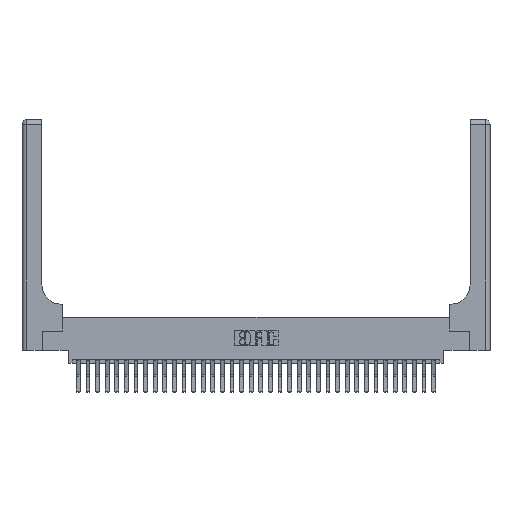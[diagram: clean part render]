
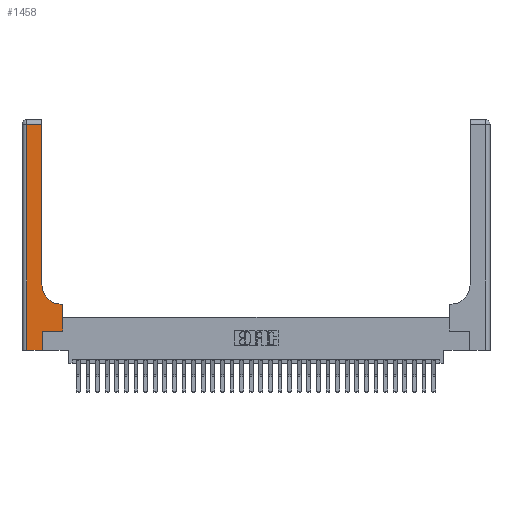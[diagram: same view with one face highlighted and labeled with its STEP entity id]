
A CAD part, top view. The second image highlights one B-rep face of the part: STEP entity #1458.
In plain terms, the highlighted planar face has unit normal (0, 0, 1).
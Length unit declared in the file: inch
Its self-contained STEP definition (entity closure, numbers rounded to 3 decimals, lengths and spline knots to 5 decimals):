
#541 = LINE ( 'NONE', #20445, #6170 ) ;
#696 = EDGE_CURVE ( 'NONE', #22260, #21338, #13939, .T. ) ;
#1458 = ADVANCED_FACE ( 'NONE', ( #4975 ), #24261, .F. ) ;
#2265 = LINE ( 'NONE', #23883, #15712 ) ;
#3300 = VECTOR ( 'NONE', #7871, 39.37008 ) ;
#3541 = EDGE_CURVE ( 'NONE', #21365, #20497, #11126, .T. ) ;
#3670 = CARTESIAN_POINT ( 'NONE',  ( 0.26, 0.6, 0.37 ) ) ;
#4286 = VECTOR ( 'NONE', #17962, 39.37008 ) ;
#4975 = FACE_OUTER_BOUND ( 'NONE', #5964, .T. ) ;
#5019 = CARTESIAN_POINT ( 'NONE',  ( 0.265, 0.25, 0.37 ) ) ;
#5042 = CARTESIAN_POINT ( 'NONE',  ( 0.26, 0.85, 0.37 ) ) ;
#5317 = VECTOR ( 'NONE', #6080, 39.37008 ) ;
#5964 = EDGE_LOOP ( 'NONE', ( #6043, #12499, #15227, #9542, #11145, #26538, #6670, #25798, #25762 ) ) ;
#6043 = ORIENTED_EDGE ( 'NONE', *, *, #25653, .T. ) ;
#6080 = DIRECTION ( 'NONE',  ( 0., 1., 0. ) ) ;
#6170 = VECTOR ( 'NONE', #25178, 39.37008 ) ;
#6177 = CARTESIAN_POINT ( 'NONE',  ( 0.528, 0.25, 0.37 ) ) ;
#6528 = CIRCLE ( 'NONE', #27535, 0.25 ) ;
#6670 = ORIENTED_EDGE ( 'NONE', *, *, #21326, .T. ) ;
#7767 = DIRECTION ( 'NONE',  ( 0., 0., -1. ) ) ;
#7871 = DIRECTION ( 'NONE',  ( 1., 0., 0. ) ) ;
#8234 = EDGE_CURVE ( 'NONE', #17478, #21365, #10504, .T. ) ;
#8480 = CARTESIAN_POINT ( 'NONE',  ( 0.528, 0.25, 0.37 ) ) ;
#9542 = ORIENTED_EDGE ( 'NONE', *, *, #3541, .T. ) ;
#9939 = CARTESIAN_POINT ( 'NONE',  ( 0.51, 0.85, 0.37 ) ) ;
#10181 = EDGE_CURVE ( 'NONE', #20497, #22260, #29548, .T. ) ;
#10287 = CARTESIAN_POINT ( 'NONE',  ( 0.06, 3., 0.37 ) ) ;
#10504 = LINE ( 'NONE', #10287, #22388 ) ;
#11126 = LINE ( 'NONE', #26641, #3300 ) ;
#11145 = ORIENTED_EDGE ( 'NONE', *, *, #10181, .T. ) ;
#11158 = EDGE_CURVE ( 'NONE', #27745, #24170, #12113, .T. ) ;
#12113 = LINE ( 'NONE', #3670, #4286 ) ;
#12315 = DIRECTION ( 'NONE',  ( 1., 0., 0. ) ) ;
#12389 = LINE ( 'NONE', #8480, #5317 ) ;
#12450 = VECTOR ( 'NONE', #21523, 39.37008 ) ;
#12499 = ORIENTED_EDGE ( 'NONE', *, *, #19360, .T. ) ;
#12671 = DIRECTION ( 'NONE',  ( 0., -1., 0. ) ) ;
#13864 = VERTEX_POINT ( 'NONE', #5042 ) ;
#13939 = LINE ( 'NONE', #5019, #12450 ) ;
#14463 = CARTESIAN_POINT ( 'NONE',  ( 0.265, 0., 0.37 ) ) ;
#15227 = ORIENTED_EDGE ( 'NONE', *, *, #8234, .T. ) ;
#15712 = VECTOR ( 'NONE', #26257, 39.37008 ) ;
#16198 = AXIS2_PLACEMENT_3D ( 'NONE', #19641, #7767, #24358 ) ;
#17478 = VERTEX_POINT ( 'NONE', #19464 ) ;
#17962 = DIRECTION ( 'NONE',  ( -1., 0., 0. ) ) ;
#19262 = DIRECTION ( 'NONE',  ( 0., 1., 0. ) ) ;
#19360 = EDGE_CURVE ( 'NONE', #23771, #17478, #541, .T. ) ;
#19464 = CARTESIAN_POINT ( 'NONE',  ( 0.06, 2.94, 0.37 ) ) ;
#19638 = EDGE_CURVE ( 'NONE', #24170, #13864, #6528, .T. ) ;
#19641 = CARTESIAN_POINT ( 'NONE',  ( 0., 3., 0.37 ) ) ;
#20445 = CARTESIAN_POINT ( 'NONE',  ( 0., 2.94, 0.37 ) ) ;
#20497 = VERTEX_POINT ( 'NONE', #22208 ) ;
#21326 = EDGE_CURVE ( 'NONE', #21338, #27745, #12389, .T. ) ;
#21338 = VERTEX_POINT ( 'NONE', #6177 ) ;
#21365 = VERTEX_POINT ( 'NONE', #22784 ) ;
#21523 = DIRECTION ( 'NONE',  ( 1., 0., 0. ) ) ;
#22208 = CARTESIAN_POINT ( 'NONE',  ( 0.265, 0., 0.37 ) ) ;
#22260 = VERTEX_POINT ( 'NONE', #30483 ) ;
#22388 = VECTOR ( 'NONE', #12671, 39.37008 ) ;
#22503 = CARTESIAN_POINT ( 'NONE',  ( 0.51, 0.6, 0.37 ) ) ;
#22784 = CARTESIAN_POINT ( 'NONE',  ( 0.06, 0., 0.37 ) ) ;
#23771 = VERTEX_POINT ( 'NONE', #28007 ) ;
#23883 = CARTESIAN_POINT ( 'NONE',  ( 0.26, 3., 0.37 ) ) ;
#24170 = VERTEX_POINT ( 'NONE', #22503 ) ;
#24261 = PLANE ( 'NONE',  #16198 ) ;
#24358 = DIRECTION ( 'NONE',  ( -1., 0., 0. ) ) ;
#25178 = DIRECTION ( 'NONE',  ( -1., 0., 0. ) ) ;
#25653 = EDGE_CURVE ( 'NONE', #13864, #23771, #2265, .T. ) ;
#25762 = ORIENTED_EDGE ( 'NONE', *, *, #19638, .T. ) ;
#25798 = ORIENTED_EDGE ( 'NONE', *, *, #11158, .T. ) ;
#26257 = DIRECTION ( 'NONE',  ( 0., 1., 0. ) ) ;
#26510 = DIRECTION ( 'NONE',  ( 0., 0., -1. ) ) ;
#26538 = ORIENTED_EDGE ( 'NONE', *, *, #696, .T. ) ;
#26641 = CARTESIAN_POINT ( 'NONE',  ( 0., 0., 0.37 ) ) ;
#27535 = AXIS2_PLACEMENT_3D ( 'NONE', #9939, #26510, #12315 ) ;
#27745 = VERTEX_POINT ( 'NONE', #30205 ) ;
#28007 = CARTESIAN_POINT ( 'NONE',  ( 0.26, 2.94, 0.37 ) ) ;
#29548 = LINE ( 'NONE', #14463, #30313 ) ;
#30205 = CARTESIAN_POINT ( 'NONE',  ( 0.528, 0.6, 0.37 ) ) ;
#30313 = VECTOR ( 'NONE', #19262, 39.37008 ) ;
#30483 = CARTESIAN_POINT ( 'NONE',  ( 0.265, 0.25, 0.37 ) ) ;
